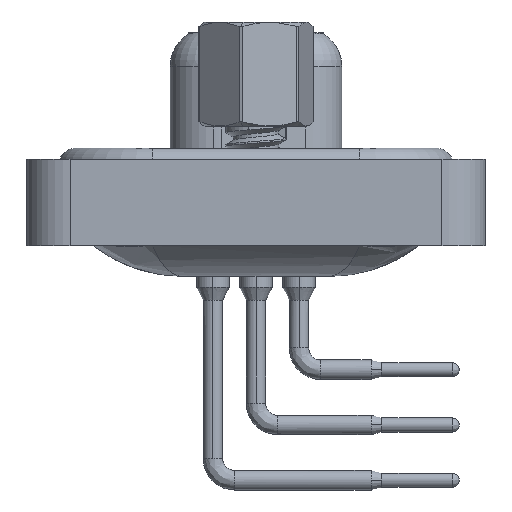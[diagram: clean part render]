
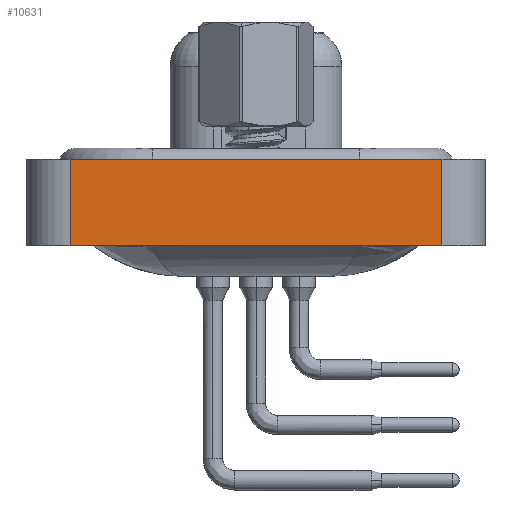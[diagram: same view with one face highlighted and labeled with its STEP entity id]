
A CAD part, left-side view. The second image highlights one B-rep face of the part: STEP entity #10631.
In plain terms, the highlighted planar face has unit normal (-1, 0, 0).
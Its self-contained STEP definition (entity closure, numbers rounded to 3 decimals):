
#605 = CARTESIAN_POINT ( 'NONE',  ( -7.26, 8.55, -3.6 ) ) ;
#970 = EDGE_CURVE ( 'NONE', #20751, #16977, #22991, .T. ) ;
#1344 = DIRECTION ( 'NONE',  ( 0., 0., 1. ) ) ;
#1931 = CARTESIAN_POINT ( 'NONE',  ( -7.26, -8.55, -3.6 ) ) ;
#2346 = CARTESIAN_POINT ( 'NONE',  ( -7.26, -8.55, 0.4 ) ) ;
#2495 = EDGE_CURVE ( 'NONE', #5467, #22720, #19124, .T. ) ;
#3046 = EDGE_LOOP ( 'NONE', ( #17361, #9182, #24144, #9260 ) ) ;
#3199 = DIRECTION ( 'NONE',  ( -1., 0., 0. ) ) ;
#5008 = FACE_OUTER_BOUND ( 'NONE', #3046, .T. ) ;
#5467 = VERTEX_POINT ( 'NONE', #5651 ) ;
#5651 = CARTESIAN_POINT ( 'NONE',  ( -7.26, 8.55, -3.6 ) ) ;
#6367 = LINE ( 'NONE', #2346, #18812 ) ;
#6896 = CARTESIAN_POINT ( 'NONE',  ( -7.26, 8.55, 0.4 ) ) ;
#7163 = CARTESIAN_POINT ( 'NONE',  ( -7.26, -8.55, -3.6 ) ) ;
#7898 = VECTOR ( 'NONE', #16775, 1000. ) ;
#8303 = CARTESIAN_POINT ( 'NONE',  ( -7.26, -8.55, -3.6 ) ) ;
#8910 = CARTESIAN_POINT ( 'NONE',  ( -7.26, -8.55, -3.6 ) ) ;
#9182 = ORIENTED_EDGE ( 'NONE', *, *, #18885, .F. ) ;
#9260 = ORIENTED_EDGE ( 'NONE', *, *, #13436, .T. ) ;
#10631 = ADVANCED_FACE ( 'NONE', ( #5008 ), #11257, .T. ) ;
#11257 = PLANE ( 'NONE',  #15136 ) ;
#13436 = EDGE_CURVE ( 'NONE', #5467, #20751, #14157, .T. ) ;
#14157 = LINE ( 'NONE', #8303, #19037 ) ;
#14270 = DIRECTION ( 'NONE',  ( 0., -1., 0. ) ) ;
#15136 = AXIS2_PLACEMENT_3D ( 'NONE', #8910, #3199, #17088 ) ;
#16775 = DIRECTION ( 'NONE',  ( 0., 0., 1. ) ) ;
#16977 = VERTEX_POINT ( 'NONE', #22193 ) ;
#17088 = DIRECTION ( 'NONE',  ( 0., 0., 1. ) ) ;
#17361 = ORIENTED_EDGE ( 'NONE', *, *, #970, .T. ) ;
#18812 = VECTOR ( 'NONE', #20384, 1000. ) ;
#18885 = EDGE_CURVE ( 'NONE', #22720, #16977, #6367, .T. ) ;
#19037 = VECTOR ( 'NONE', #14270, 1000. ) ;
#19124 = LINE ( 'NONE', #605, #21026 ) ;
#20384 = DIRECTION ( 'NONE',  ( 0., -1., 0. ) ) ;
#20751 = VERTEX_POINT ( 'NONE', #1931 ) ;
#21026 = VECTOR ( 'NONE', #1344, 1000. ) ;
#22193 = CARTESIAN_POINT ( 'NONE',  ( -7.26, -8.55, 0.4 ) ) ;
#22720 = VERTEX_POINT ( 'NONE', #6896 ) ;
#22991 = LINE ( 'NONE', #7163, #7898 ) ;
#24144 = ORIENTED_EDGE ( 'NONE', *, *, #2495, .F. ) ;
